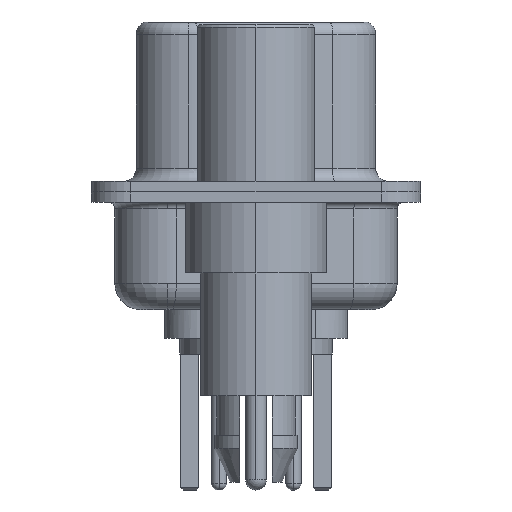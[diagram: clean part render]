
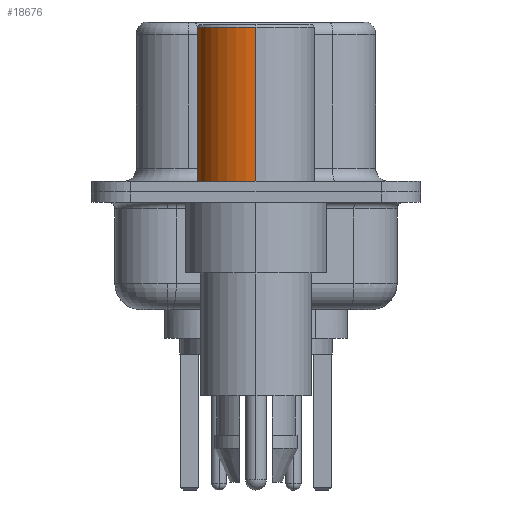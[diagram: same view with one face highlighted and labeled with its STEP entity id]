
A CAD part, left-side view. The second image highlights one B-rep face of the part: STEP entity #18676.
In plain terms, the highlighted cylindrical face has radius 2.25 mm (diameter 4.5 mm), a partial arc.
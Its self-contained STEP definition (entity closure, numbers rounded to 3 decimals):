
#172 = DIRECTION ( 'NONE',  ( 0., 0., 1. ) ) ;
#1137 = DIRECTION ( 'NONE',  ( 0., 0., 1. ) ) ;
#1442 = EDGE_CURVE ( 'NONE', #3556, #2452, #11086, .T. ) ;
#1663 = CARTESIAN_POINT ( 'NONE',  ( 0., 0., 0.581 ) ) ;
#1673 = CARTESIAN_POINT ( 'NONE',  ( 0., 0., 0.4 ) ) ;
#2452 = VERTEX_POINT ( 'NONE', #5097 ) ;
#3464 = CARTESIAN_POINT ( 'NONE',  ( 0., 0., 6.3 ) ) ;
#3556 = VERTEX_POINT ( 'NONE', #13834 ) ;
#4422 = CARTESIAN_POINT ( 'NONE',  ( 2.25, 0., 0.581 ) ) ;
#5097 = CARTESIAN_POINT ( 'NONE',  ( -2.25, 0., 0.4 ) ) ;
#5314 = LINE ( 'NONE', #4422, #19146 ) ;
#5430 = DIRECTION ( 'NONE',  ( 0., 0., 1. ) ) ;
#5506 = CYLINDRICAL_SURFACE ( 'NONE', #17760, 2.25 ) ;
#5925 = ORIENTED_EDGE ( 'NONE', *, *, #15992, .T. ) ;
#6066 = CARTESIAN_POINT ( 'NONE',  ( -2.25, 0., 6.3 ) ) ;
#7498 = VECTOR ( 'NONE', #1137, 1000. ) ;
#7797 = CARTESIAN_POINT ( 'NONE',  ( 2.25, 0., 6.3 ) ) ;
#8904 = VERTEX_POINT ( 'NONE', #7797 ) ;
#10236 = DIRECTION ( 'NONE',  ( 1., 0., 0. ) ) ;
#10295 = DIRECTION ( 'NONE',  ( 1., 0., 0. ) ) ;
#11086 = CIRCLE ( 'NONE', #13768, 2.25 ) ;
#11303 = LINE ( 'NONE', #20128, #7498 ) ;
#11438 = ORIENTED_EDGE ( 'NONE', *, *, #18280, .F. ) ;
#12187 = DIRECTION ( 'NONE',  ( 1., 0., 0. ) ) ;
#12314 = ORIENTED_EDGE ( 'NONE', *, *, #15272, .F. ) ;
#13768 = AXIS2_PLACEMENT_3D ( 'NONE', #1673, #172, #12187 ) ;
#13834 = CARTESIAN_POINT ( 'NONE',  ( 2.25, 0., 0.4 ) ) ;
#14463 = FACE_OUTER_BOUND ( 'NONE', #16333, .T. ) ;
#15252 = AXIS2_PLACEMENT_3D ( 'NONE', #3464, #5430, #10236 ) ;
#15272 = EDGE_CURVE ( 'NONE', #3556, #8904, #5314, .T. ) ;
#15568 = CIRCLE ( 'NONE', #15252, 2.25 ) ;
#15992 = EDGE_CURVE ( 'NONE', #2452, #21387, #11303, .T. ) ;
#16333 = EDGE_LOOP ( 'NONE', ( #19551, #5925, #11438, #12314 ) ) ;
#16599 = DIRECTION ( 'NONE',  ( 0., 0., 1. ) ) ;
#17760 = AXIS2_PLACEMENT_3D ( 'NONE', #1663, #22448, #10295 ) ;
#18280 = EDGE_CURVE ( 'NONE', #8904, #21387, #15568, .T. ) ;
#18676 = ADVANCED_FACE ( 'NONE', ( #14463 ), #5506, .T. ) ;
#19146 = VECTOR ( 'NONE', #16599, 1000. ) ;
#19551 = ORIENTED_EDGE ( 'NONE', *, *, #1442, .T. ) ;
#20128 = CARTESIAN_POINT ( 'NONE',  ( -2.25, 0., 0.581 ) ) ;
#21387 = VERTEX_POINT ( 'NONE', #6066 ) ;
#22448 = DIRECTION ( 'NONE',  ( 0., 0., 1. ) ) ;
